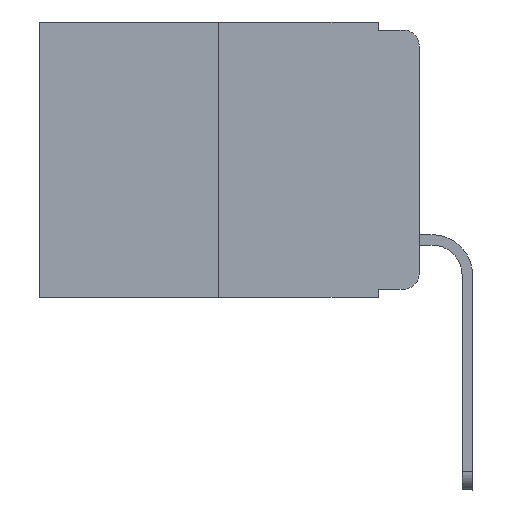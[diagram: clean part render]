
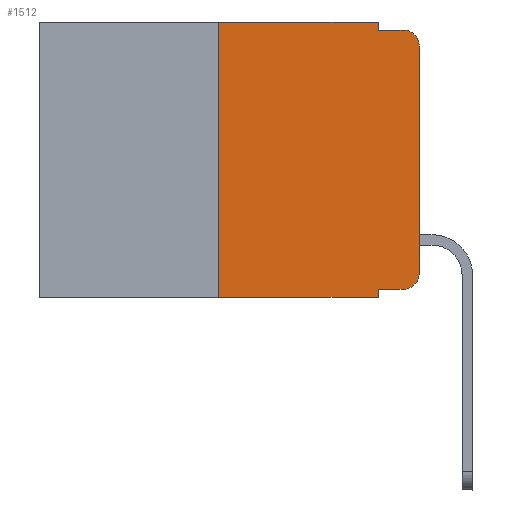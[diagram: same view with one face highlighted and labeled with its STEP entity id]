
A CAD part, left-side view. The second image highlights one B-rep face of the part: STEP entity #1512.
In plain terms, the highlighted planar face has unit normal (-1, 0, 0).
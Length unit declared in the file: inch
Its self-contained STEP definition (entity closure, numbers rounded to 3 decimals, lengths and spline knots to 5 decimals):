
#14 = ORIENTED_EDGE ( 'NONE', *, *, #7828, .F. ) ;
#213 = ORIENTED_EDGE ( 'NONE', *, *, #12736, .F. ) ;
#809 = EDGE_CURVE ( 'NONE', #21410, #4803, #4664, .T. ) ;
#925 = LINE ( 'NONE', #22537, #7457 ) ;
#956 = DIRECTION ( 'NONE',  ( 0., -1., 0. ) ) ;
#1287 = EDGE_CURVE ( 'NONE', #15043, #11100, #6374, .T. ) ;
#1322 = DIRECTION ( 'NONE',  ( 0., 0., 1. ) ) ;
#1512 = ADVANCED_FACE ( 'NONE', ( #20732 ), #24637, .F. ) ;
#1532 = CARTESIAN_POINT ( 'NONE',  ( 0., 0.051, -0.343 ) ) ;
#1555 = LINE ( 'NONE', #1812, #8385 ) ;
#1812 = CARTESIAN_POINT ( 'NONE',  ( 0., 0.051, -0.333 ) ) ;
#1863 = CARTESIAN_POINT ( 'NONE',  ( 0., 0., 0. ) ) ;
#2271 = AXIS2_PLACEMENT_3D ( 'NONE', #7168, #17009, #5235 ) ;
#3270 = CARTESIAN_POINT ( 'NONE',  ( 0., 0.25, 0. ) ) ;
#4137 = ORIENTED_EDGE ( 'NONE', *, *, #9009, .F. ) ;
#4191 = EDGE_CURVE ( 'NONE', #5312, #18418, #20991, .T. ) ;
#4454 = DIRECTION ( 'NONE',  ( 0., 0., -1. ) ) ;
#4664 = CIRCLE ( 'NONE', #16678, 0.02 ) ;
#4803 = VERTEX_POINT ( 'NONE', #14782 ) ;
#4909 = CARTESIAN_POINT ( 'NONE',  ( 0., 0.051, -0.333 ) ) ;
#4965 = LINE ( 'NONE', #12889, #18263 ) ;
#5235 = DIRECTION ( 'NONE',  ( 0., 0., -1. ) ) ;
#5312 = VERTEX_POINT ( 'NONE', #10715 ) ;
#5740 = DIRECTION ( 'NONE',  ( 0., 0., 1. ) ) ;
#5939 = VECTOR ( 'NONE', #22807, 39.37008 ) ;
#6167 = CARTESIAN_POINT ( 'NONE',  ( 0., 0.051, 0. ) ) ;
#6201 = CARTESIAN_POINT ( 'NONE',  ( 0., 0.051, -0.01 ) ) ;
#6258 = CARTESIAN_POINT ( 'NONE',  ( 0., 0.02, -0.313 ) ) ;
#6290 = CARTESIAN_POINT ( 'NONE',  ( 0., 0.051, 0. ) ) ;
#6342 = CARTESIAN_POINT ( 'NONE',  ( 0., 0.051, -0.01 ) ) ;
#6344 = VECTOR ( 'NONE', #1322, 39.37008 ) ;
#6374 = CIRCLE ( 'NONE', #10970, 0.02 ) ;
#6850 = EDGE_LOOP ( 'NONE', ( #19400, #22403, #14, #213, #4137, #10748, #13555, #19790, #7325, #15346 ) ) ;
#6897 = DIRECTION ( 'NONE',  ( 0., -1., 0. ) ) ;
#7168 = CARTESIAN_POINT ( 'NONE',  ( 0., 0.473, 0. ) ) ;
#7325 = ORIENTED_EDGE ( 'NONE', *, *, #13274, .T. ) ;
#7457 = VECTOR ( 'NONE', #6897, 39.37008 ) ;
#7828 = EDGE_CURVE ( 'NONE', #13459, #4803, #18382, .T. ) ;
#7972 = CARTESIAN_POINT ( 'NONE',  ( 0., 0., -0.313 ) ) ;
#8246 = DIRECTION ( 'NONE',  ( -1., 0., 0. ) ) ;
#8385 = VECTOR ( 'NONE', #9738, 39.37008 ) ;
#9009 = EDGE_CURVE ( 'NONE', #18418, #9526, #925, .T. ) ;
#9526 = VERTEX_POINT ( 'NONE', #6290 ) ;
#9738 = DIRECTION ( 'NONE',  ( 0., -1., 0. ) ) ;
#10292 = DIRECTION ( 'NONE',  ( -1., 0., 0. ) ) ;
#10715 = CARTESIAN_POINT ( 'NONE',  ( 0., 0.25, -0.343 ) ) ;
#10748 = ORIENTED_EDGE ( 'NONE', *, *, #4191, .F. ) ;
#10903 = VECTOR ( 'NONE', #5740, 39.37008 ) ;
#10960 = LINE ( 'NONE', #14962, #5939 ) ;
#10970 = AXIS2_PLACEMENT_3D ( 'NONE', #6258, #10292, #4454 ) ;
#11100 = VERTEX_POINT ( 'NONE', #7972 ) ;
#11654 = VECTOR ( 'NONE', #14097, 39.37008 ) ;
#12736 = EDGE_CURVE ( 'NONE', #9526, #13459, #10960, .T. ) ;
#12889 = CARTESIAN_POINT ( 'NONE',  ( 0., 0.473, -0.343 ) ) ;
#13274 = EDGE_CURVE ( 'NONE', #22159, #15043, #1555, .T. ) ;
#13459 = VERTEX_POINT ( 'NONE', #6342 ) ;
#13555 = ORIENTED_EDGE ( 'NONE', *, *, #15997, .T. ) ;
#14030 = EDGE_CURVE ( 'NONE', #22159, #16496, #17969, .T. ) ;
#14097 = DIRECTION ( 'NONE',  ( 0., 0., -1. ) ) ;
#14782 = CARTESIAN_POINT ( 'NONE',  ( 0., 0.02, -0.01 ) ) ;
#14962 = CARTESIAN_POINT ( 'NONE',  ( 0., 0.051, 0. ) ) ;
#15043 = VERTEX_POINT ( 'NONE', #16451 ) ;
#15346 = ORIENTED_EDGE ( 'NONE', *, *, #1287, .T. ) ;
#15997 = EDGE_CURVE ( 'NONE', #5312, #16496, #4965, .T. ) ;
#16451 = CARTESIAN_POINT ( 'NONE',  ( 0., 0.02, -0.333 ) ) ;
#16496 = VERTEX_POINT ( 'NONE', #1532 ) ;
#16678 = AXIS2_PLACEMENT_3D ( 'NONE', #22453, #8246, #22312 ) ;
#17009 = DIRECTION ( 'NONE',  ( 1., 0., 0. ) ) ;
#17353 = EDGE_CURVE ( 'NONE', #11100, #21410, #25522, .T. ) ;
#17969 = LINE ( 'NONE', #6167, #11654 ) ;
#18242 = DIRECTION ( 'NONE',  ( 0., -1., 0. ) ) ;
#18263 = VECTOR ( 'NONE', #956, 39.37008 ) ;
#18382 = LINE ( 'NONE', #6201, #21857 ) ;
#18418 = VERTEX_POINT ( 'NONE', #22291 ) ;
#19400 = ORIENTED_EDGE ( 'NONE', *, *, #17353, .T. ) ;
#19790 = ORIENTED_EDGE ( 'NONE', *, *, #14030, .F. ) ;
#20732 = FACE_OUTER_BOUND ( 'NONE', #6850, .T. ) ;
#20991 = LINE ( 'NONE', #3270, #6344 ) ;
#21410 = VERTEX_POINT ( 'NONE', #25523 ) ;
#21857 = VECTOR ( 'NONE', #18242, 39.37008 ) ;
#22159 = VERTEX_POINT ( 'NONE', #4909 ) ;
#22291 = CARTESIAN_POINT ( 'NONE',  ( 0., 0.25, 0. ) ) ;
#22312 = DIRECTION ( 'NONE',  ( 0., 0., -1. ) ) ;
#22403 = ORIENTED_EDGE ( 'NONE', *, *, #809, .T. ) ;
#22453 = CARTESIAN_POINT ( 'NONE',  ( 0., 0.02, -0.03 ) ) ;
#22537 = CARTESIAN_POINT ( 'NONE',  ( 0., 0.473, 0. ) ) ;
#22807 = DIRECTION ( 'NONE',  ( 0., 0., -1. ) ) ;
#24637 = PLANE ( 'NONE',  #2271 ) ;
#25522 = LINE ( 'NONE', #1863, #10903 ) ;
#25523 = CARTESIAN_POINT ( 'NONE',  ( 0., 0., -0.03 ) ) ;
